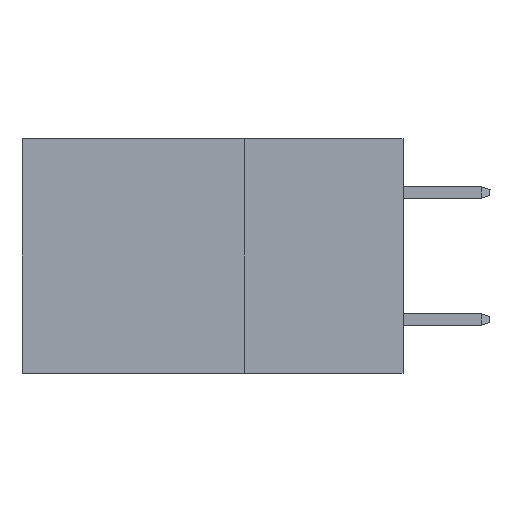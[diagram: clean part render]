
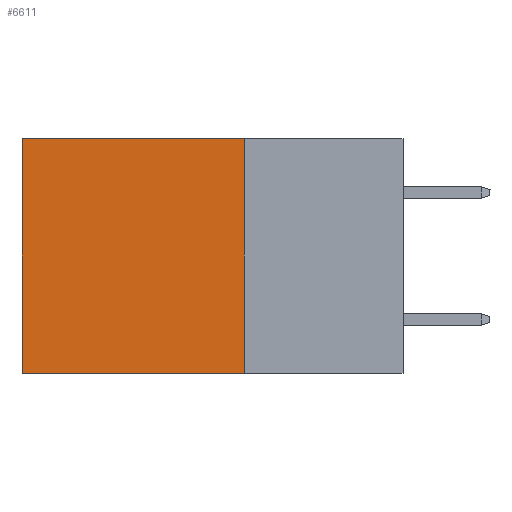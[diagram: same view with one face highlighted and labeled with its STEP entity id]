
A CAD part, left-side view. The second image highlights one B-rep face of the part: STEP entity #6611.
In plain terms, the highlighted planar face has unit normal (-1, 0, 0).
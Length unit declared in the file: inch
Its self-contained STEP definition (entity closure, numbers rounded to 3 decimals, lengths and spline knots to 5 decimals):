
#1732 = EDGE_CURVE ( 'NONE', #10409, #16220, #3878, .T. ) ;
#2113 = DIRECTION ( 'NONE',  ( 0., 1., 0. ) ) ;
#3039 = LINE ( 'NONE', #18170, #7538 ) ;
#3878 = LINE ( 'NONE', #16472, #12569 ) ;
#4727 = DIRECTION ( 'NONE',  ( 0., 0., -1. ) ) ;
#4852 = EDGE_CURVE ( 'NONE', #7417, #10265, #9353, .T. ) ;
#5720 = DIRECTION ( 'NONE',  ( 1., 0., 0. ) ) ;
#5951 = ORIENTED_EDGE ( 'NONE', *, *, #19124, .T. ) ;
#6611 = ADVANCED_FACE ( 'NONE', ( #14886 ), #7532, .F. ) ;
#6647 = LINE ( 'NONE', #17438, #7554 ) ;
#7021 = CARTESIAN_POINT ( 'NONE',  ( 0.2875, 0.25, 0. ) ) ;
#7417 = VERTEX_POINT ( 'NONE', #12046 ) ;
#7532 = PLANE ( 'NONE',  #11773 ) ;
#7538 = VECTOR ( 'NONE', #15336, 39.37008 ) ;
#7554 = VECTOR ( 'NONE', #2113, 39.37008 ) ;
#7905 = ORIENTED_EDGE ( 'NONE', *, *, #1732, .F. ) ;
#9256 = CARTESIAN_POINT ( 'NONE',  ( 0.2875, 0.6, 0. ) ) ;
#9353 = LINE ( 'NONE', #9256, #18613 ) ;
#9637 = EDGE_LOOP ( 'NONE', ( #11545, #16744, #7905, #5951 ) ) ;
#10265 = VERTEX_POINT ( 'NONE', #18930 ) ;
#10409 = VERTEX_POINT ( 'NONE', #7021 ) ;
#10453 = DIRECTION ( 'NONE',  ( 0., 0., -1. ) ) ;
#11469 = CARTESIAN_POINT ( 'NONE',  ( 0.2875, 0.25, -0.37 ) ) ;
#11545 = ORIENTED_EDGE ( 'NONE', *, *, #4852, .T. ) ;
#11773 = AXIS2_PLACEMENT_3D ( 'NONE', #13370, #5720, #10453 ) ;
#12046 = CARTESIAN_POINT ( 'NONE',  ( 0.2875, 0.6, 0. ) ) ;
#12569 = VECTOR ( 'NONE', #15172, 39.37008 ) ;
#13370 = CARTESIAN_POINT ( 'NONE',  ( 0.2875, 0.25, 0. ) ) ;
#14886 = FACE_OUTER_BOUND ( 'NONE', #9637, .T. ) ;
#15172 = DIRECTION ( 'NONE',  ( 0., 0., -1. ) ) ;
#15336 = DIRECTION ( 'NONE',  ( 0., 1., 0. ) ) ;
#16220 = VERTEX_POINT ( 'NONE', #11469 ) ;
#16472 = CARTESIAN_POINT ( 'NONE',  ( 0.2875, 0.25, 0. ) ) ;
#16744 = ORIENTED_EDGE ( 'NONE', *, *, #18013, .F. ) ;
#17438 = CARTESIAN_POINT ( 'NONE',  ( 0.2875, 0.25, -0.37 ) ) ;
#18013 = EDGE_CURVE ( 'NONE', #16220, #10265, #6647, .T. ) ;
#18170 = CARTESIAN_POINT ( 'NONE',  ( 0.2875, 0.25, 0. ) ) ;
#18613 = VECTOR ( 'NONE', #4727, 39.37008 ) ;
#18930 = CARTESIAN_POINT ( 'NONE',  ( 0.2875, 0.6, -0.37 ) ) ;
#19124 = EDGE_CURVE ( 'NONE', #10409, #7417, #3039, .T. ) ;
